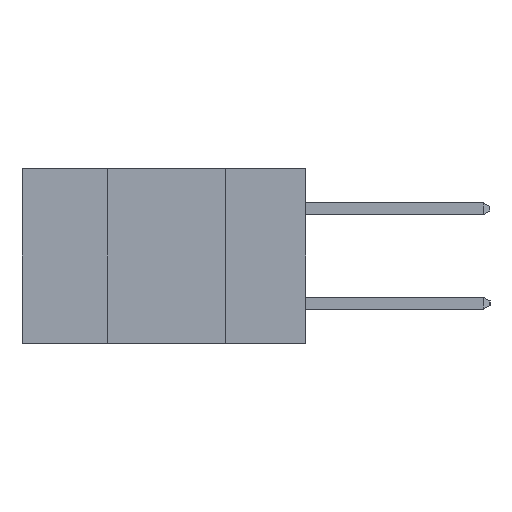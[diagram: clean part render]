
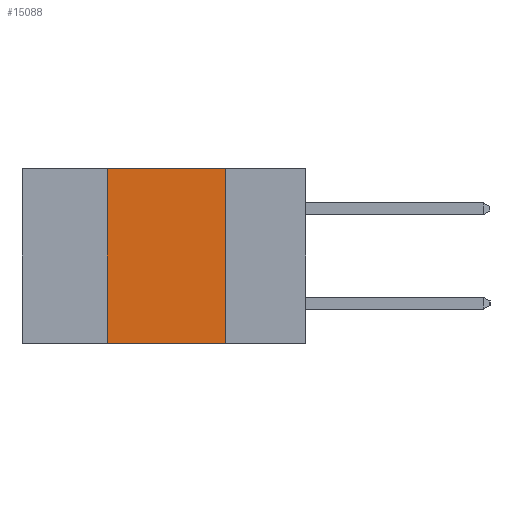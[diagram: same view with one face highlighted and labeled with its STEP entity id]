
A CAD part, left-side view. The second image highlights one B-rep face of the part: STEP entity #15088.
In plain terms, the highlighted planar face has unit normal (-1, 0, 0).
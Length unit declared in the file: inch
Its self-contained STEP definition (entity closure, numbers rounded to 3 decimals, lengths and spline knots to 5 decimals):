
#1354 = EDGE_LOOP ( 'NONE', ( #6999, #15518, #16452, #13878 ) ) ;
#1691 = CARTESIAN_POINT ( 'NONE',  ( 0., 0.17, -0.37 ) ) ;
#2984 = DIRECTION ( 'NONE',  ( 1., 0., 0. ) ) ;
#3335 = DIRECTION ( 'NONE',  ( 0., 0., 1. ) ) ;
#5496 = VERTEX_POINT ( 'NONE', #15064 ) ;
#6718 = CARTESIAN_POINT ( 'NONE',  ( 0., 0.6, 0. ) ) ;
#6742 = CARTESIAN_POINT ( 'NONE',  ( 0., 0.17, -0.37 ) ) ;
#6807 = LINE ( 'NONE', #6718, #18823 ) ;
#6999 = ORIENTED_EDGE ( 'NONE', *, *, #18594, .F. ) ;
#7448 = LINE ( 'NONE', #1691, #11439 ) ;
#7622 = FACE_OUTER_BOUND ( 'NONE', #1354, .T. ) ;
#8212 = CARTESIAN_POINT ( 'NONE',  ( 0., 0.42, -0.37 ) ) ;
#8591 = LINE ( 'NONE', #12405, #16626 ) ;
#8730 = DIRECTION ( 'NONE',  ( 0., -1., 0. ) ) ;
#9054 = CARTESIAN_POINT ( 'NONE',  ( 0., 0.42, 0. ) ) ;
#11439 = VECTOR ( 'NONE', #12313, 39.37008 ) ;
#11716 = LINE ( 'NONE', #17767, #15744 ) ;
#12313 = DIRECTION ( 'NONE',  ( 0., 0., -1. ) ) ;
#12405 = CARTESIAN_POINT ( 'NONE',  ( 0., 0.42, -0.37 ) ) ;
#13296 = AXIS2_PLACEMENT_3D ( 'NONE', #19526, #2984, #13588 ) ;
#13588 = DIRECTION ( 'NONE',  ( 0., 0., -1. ) ) ;
#13589 = EDGE_CURVE ( 'NONE', #15103, #18860, #11716, .T. ) ;
#13878 = ORIENTED_EDGE ( 'NONE', *, *, #13589, .T. ) ;
#14604 = EDGE_CURVE ( 'NONE', #15103, #18498, #8591, .T. ) ;
#15064 = CARTESIAN_POINT ( 'NONE',  ( 0., 0.17, 0. ) ) ;
#15088 = ADVANCED_FACE ( 'NONE', ( #7622 ), #18045, .F. ) ;
#15103 = VERTEX_POINT ( 'NONE', #8212 ) ;
#15518 = ORIENTED_EDGE ( 'NONE', *, *, #17600, .F. ) ;
#15744 = VECTOR ( 'NONE', #8730, 39.37008 ) ;
#16452 = ORIENTED_EDGE ( 'NONE', *, *, #14604, .F. ) ;
#16626 = VECTOR ( 'NONE', #3335, 39.37008 ) ;
#17600 = EDGE_CURVE ( 'NONE', #18498, #5496, #6807, .T. ) ;
#17767 = CARTESIAN_POINT ( 'NONE',  ( 0., 0.6, -0.37 ) ) ;
#18045 = PLANE ( 'NONE',  #13296 ) ;
#18498 = VERTEX_POINT ( 'NONE', #9054 ) ;
#18594 = EDGE_CURVE ( 'NONE', #5496, #18860, #7448, .T. ) ;
#18764 = DIRECTION ( 'NONE',  ( 0., -1., 0. ) ) ;
#18823 = VECTOR ( 'NONE', #18764, 39.37008 ) ;
#18860 = VERTEX_POINT ( 'NONE', #6742 ) ;
#19526 = CARTESIAN_POINT ( 'NONE',  ( 0., 0.6, 0. ) ) ;
